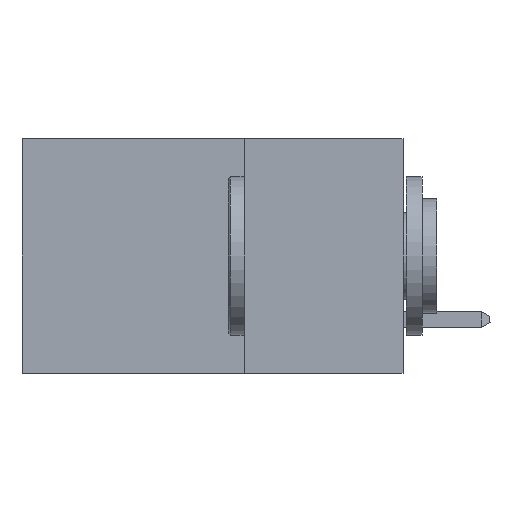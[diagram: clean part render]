
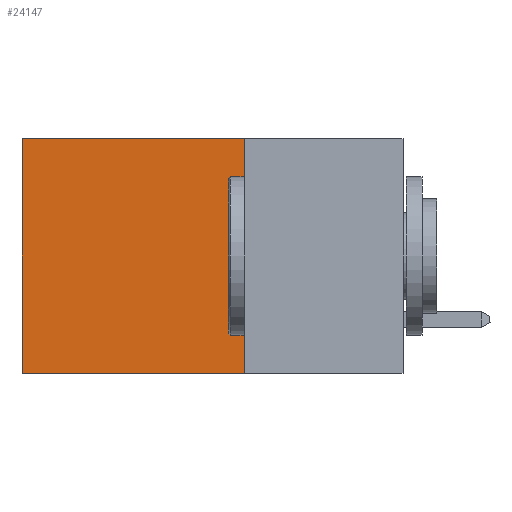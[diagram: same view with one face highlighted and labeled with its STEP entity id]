
A CAD part, left-side view. The second image highlights one B-rep face of the part: STEP entity #24147.
In plain terms, the highlighted planar face has unit normal (-1, 0, 0).
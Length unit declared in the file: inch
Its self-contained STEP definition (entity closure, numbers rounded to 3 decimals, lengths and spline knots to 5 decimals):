
#1178 = EDGE_CURVE ( 'NONE', #23888, #14755, #12040, .T. ) ;
#2859 = CARTESIAN_POINT ( 'NONE',  ( 0.2875, 0.25, 0. ) ) ;
#3045 = CARTESIAN_POINT ( 'NONE',  ( 0.2875, 0.25, -0.37 ) ) ;
#5330 = ORIENTED_EDGE ( 'NONE', *, *, #18124, .F. ) ;
#5372 = CARTESIAN_POINT ( 'NONE',  ( 0.2875, 0.25, 0. ) ) ;
#6569 = LINE ( 'NONE', #18972, #15579 ) ;
#7540 = VERTEX_POINT ( 'NONE', #19784 ) ;
#7552 = VECTOR ( 'NONE', #20593, 39.37008 ) ;
#9680 = FACE_OUTER_BOUND ( 'NONE', #9806, .T. ) ;
#9806 = EDGE_LOOP ( 'NONE', ( #16262, #5330, #22071, #17329 ) ) ;
#9978 = EDGE_CURVE ( 'NONE', #7540, #23888, #13418, .T. ) ;
#12040 = LINE ( 'NONE', #14815, #20995 ) ;
#13215 = AXIS2_PLACEMENT_3D ( 'NONE', #5372, #16478, #20963 ) ;
#13418 = LINE ( 'NONE', #2859, #7552 ) ;
#14719 = DIRECTION ( 'NONE',  ( 0., 0., -1. ) ) ;
#14755 = VERTEX_POINT ( 'NONE', #16325 ) ;
#14815 = CARTESIAN_POINT ( 'NONE',  ( 0.2875, 0.6, 0. ) ) ;
#15579 = VECTOR ( 'NONE', #16688, 39.37008 ) ;
#16262 = ORIENTED_EDGE ( 'NONE', *, *, #1178, .T. ) ;
#16325 = CARTESIAN_POINT ( 'NONE',  ( 0.2875, 0.6, -0.37 ) ) ;
#16478 = DIRECTION ( 'NONE',  ( 1., 0., 0. ) ) ;
#16688 = DIRECTION ( 'NONE',  ( 0., 1., 0. ) ) ;
#17329 = ORIENTED_EDGE ( 'NONE', *, *, #9978, .T. ) ;
#17483 = EDGE_CURVE ( 'NONE', #7540, #25563, #24425, .T. ) ;
#18124 = EDGE_CURVE ( 'NONE', #25563, #14755, #6569, .T. ) ;
#18972 = CARTESIAN_POINT ( 'NONE',  ( 0.2875, 0.25, -0.37 ) ) ;
#19784 = CARTESIAN_POINT ( 'NONE',  ( 0.2875, 0.25, 0. ) ) ;
#20593 = DIRECTION ( 'NONE',  ( 0., 1., 0. ) ) ;
#20688 = CARTESIAN_POINT ( 'NONE',  ( 0.2875, 0.25, 0. ) ) ;
#20963 = DIRECTION ( 'NONE',  ( 0., 0., -1. ) ) ;
#20995 = VECTOR ( 'NONE', #14719, 39.37008 ) ;
#21064 = DIRECTION ( 'NONE',  ( 0., 0., -1. ) ) ;
#22071 = ORIENTED_EDGE ( 'NONE', *, *, #17483, .F. ) ;
#22884 = PLANE ( 'NONE',  #13215 ) ;
#23888 = VERTEX_POINT ( 'NONE', #25344 ) ;
#24147 = ADVANCED_FACE ( 'NONE', ( #9680 ), #22884, .F. ) ;
#24425 = LINE ( 'NONE', #20688, #27559 ) ;
#25344 = CARTESIAN_POINT ( 'NONE',  ( 0.2875, 0.6, 0. ) ) ;
#25563 = VERTEX_POINT ( 'NONE', #3045 ) ;
#27559 = VECTOR ( 'NONE', #21064, 39.37008 ) ;
